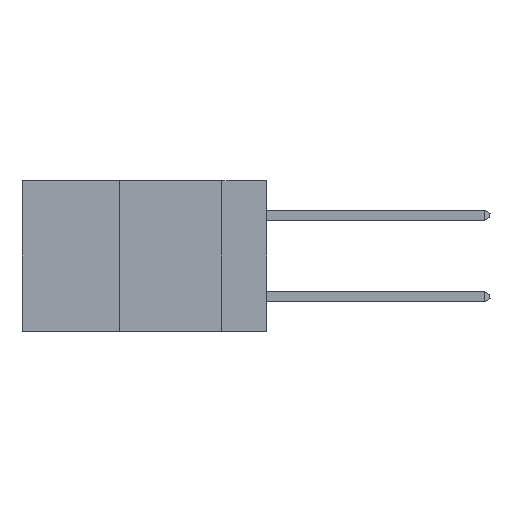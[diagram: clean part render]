
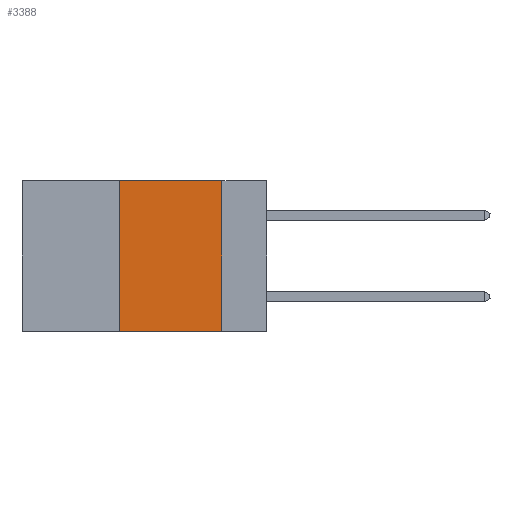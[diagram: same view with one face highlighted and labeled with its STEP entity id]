
A CAD part, left-side view. The second image highlights one B-rep face of the part: STEP entity #3388.
In plain terms, the highlighted planar face has unit normal (-1, 0, 0).
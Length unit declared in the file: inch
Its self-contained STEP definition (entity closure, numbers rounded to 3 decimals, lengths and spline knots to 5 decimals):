
#1254 = VERTEX_POINT ( 'NONE', #11551 ) ;
#1542 = ORIENTED_EDGE ( 'NONE', *, *, #29524, .F. ) ;
#3388 = ADVANCED_FACE ( 'NONE', ( #7631 ), #15018, .F. ) ;
#3913 = EDGE_LOOP ( 'NONE', ( #1542, #24474, #14270, #10921 ) ) ;
#4588 = VECTOR ( 'NONE', #6206, 39.37008 ) ;
#6206 = DIRECTION ( 'NONE',  ( 0., 0., -1. ) ) ;
#6297 = AXIS2_PLACEMENT_3D ( 'NONE', #9289, #31487, #34536 ) ;
#6941 = VECTOR ( 'NONE', #34736, 39.37008 ) ;
#7234 = LINE ( 'NONE', #25584, #4588 ) ;
#7631 = FACE_OUTER_BOUND ( 'NONE', #3913, .T. ) ;
#7814 = VERTEX_POINT ( 'NONE', #16517 ) ;
#8627 = DIRECTION ( 'NONE',  ( 0., -1., 0. ) ) ;
#9289 = CARTESIAN_POINT ( 'NONE',  ( 0., 0.6, 0. ) ) ;
#9772 = VECTOR ( 'NONE', #8627, 39.37008 ) ;
#10854 = CARTESIAN_POINT ( 'NONE',  ( 0., 0.36, 0. ) ) ;
#10921 = ORIENTED_EDGE ( 'NONE', *, *, #28344, .T. ) ;
#11551 = CARTESIAN_POINT ( 'NONE',  ( 0., 0.11, 0. ) ) ;
#14270 = ORIENTED_EDGE ( 'NONE', *, *, #29361, .F. ) ;
#15018 = PLANE ( 'NONE',  #6297 ) ;
#16517 = CARTESIAN_POINT ( 'NONE',  ( 0., 0.36, 0. ) ) ;
#17750 = VECTOR ( 'NONE', #33305, 39.37008 ) ;
#18404 = VERTEX_POINT ( 'NONE', #27412 ) ;
#18772 = LINE ( 'NONE', #31940, #6941 ) ;
#22859 = CARTESIAN_POINT ( 'NONE',  ( 0., 0.6, 0. ) ) ;
#23474 = VERTEX_POINT ( 'NONE', #32427 ) ;
#24474 = ORIENTED_EDGE ( 'NONE', *, *, #24877, .F. ) ;
#24877 = EDGE_CURVE ( 'NONE', #7814, #1254, #33475, .T. ) ;
#25584 = CARTESIAN_POINT ( 'NONE',  ( 0., 0.11, 0. ) ) ;
#27412 = CARTESIAN_POINT ( 'NONE',  ( 0., 0.36, -0.37 ) ) ;
#28344 = EDGE_CURVE ( 'NONE', #18404, #23474, #18772, .T. ) ;
#28746 = LINE ( 'NONE', #10854, #17750 ) ;
#29361 = EDGE_CURVE ( 'NONE', #18404, #7814, #28746, .T. ) ;
#29524 = EDGE_CURVE ( 'NONE', #1254, #23474, #7234, .T. ) ;
#31487 = DIRECTION ( 'NONE',  ( 1., 0., 0. ) ) ;
#31940 = CARTESIAN_POINT ( 'NONE',  ( 0., 0.6, -0.37 ) ) ;
#32427 = CARTESIAN_POINT ( 'NONE',  ( 0., 0.11, -0.37 ) ) ;
#33305 = DIRECTION ( 'NONE',  ( 0., 0., 1. ) ) ;
#33475 = LINE ( 'NONE', #22859, #9772 ) ;
#34536 = DIRECTION ( 'NONE',  ( 0., 0., -1. ) ) ;
#34736 = DIRECTION ( 'NONE',  ( 0., -1., 0. ) ) ;
